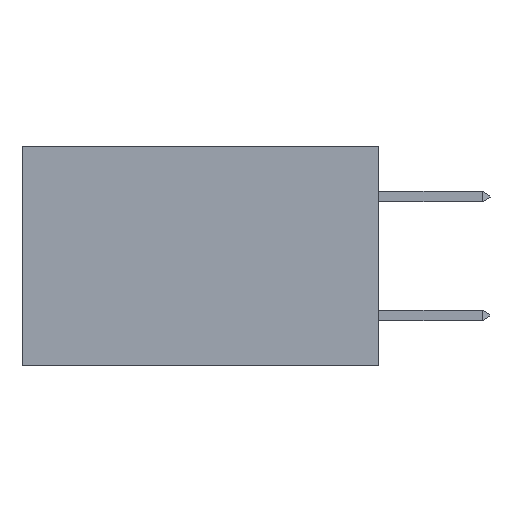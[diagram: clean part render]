
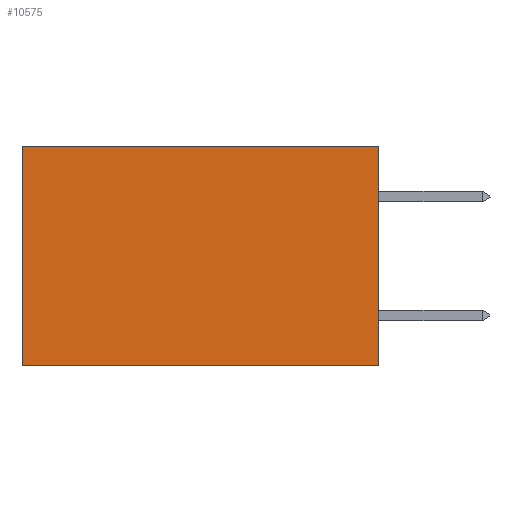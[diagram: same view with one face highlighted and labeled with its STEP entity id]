
A CAD part, left-side view. The second image highlights one B-rep face of the part: STEP entity #10575.
In plain terms, the highlighted planar face has unit normal (-1, 0, 0).
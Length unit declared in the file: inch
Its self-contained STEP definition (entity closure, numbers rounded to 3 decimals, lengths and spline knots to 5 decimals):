
#710 = ORIENTED_EDGE ( 'NONE', *, *, #22771, .F. ) ;
#1458 = VERTEX_POINT ( 'NONE', #18161 ) ;
#1689 = CARTESIAN_POINT ( 'NONE',  ( 0.2615, 0., -0.37 ) ) ;
#1898 = VERTEX_POINT ( 'NONE', #4912 ) ;
#2181 = CARTESIAN_POINT ( 'NONE',  ( 0.2615, 0., 0. ) ) ;
#3598 = LINE ( 'NONE', #21522, #13957 ) ;
#3742 = EDGE_CURVE ( 'NONE', #1898, #8556, #3598, .T. ) ;
#4210 = ORIENTED_EDGE ( 'NONE', *, *, #6669, .T. ) ;
#4297 = DIRECTION ( 'NONE',  ( 0., 1., 0. ) ) ;
#4912 = CARTESIAN_POINT ( 'NONE',  ( 0.2615, 0.6, 0. ) ) ;
#6669 = EDGE_CURVE ( 'NONE', #19979, #1898, #26027, .T. ) ;
#7958 = DIRECTION ( 'NONE',  ( 1., 0., 0. ) ) ;
#8000 = DIRECTION ( 'NONE',  ( 0., 1., 0. ) ) ;
#8039 = EDGE_LOOP ( 'NONE', ( #21949, #710, #10825, #4210 ) ) ;
#8556 = VERTEX_POINT ( 'NONE', #13973 ) ;
#8856 = VECTOR ( 'NONE', #8000, 39.37008 ) ;
#8981 = FACE_OUTER_BOUND ( 'NONE', #8039, .T. ) ;
#9508 = VECTOR ( 'NONE', #4297, 39.37008 ) ;
#10575 = ADVANCED_FACE ( 'NONE', ( #8981 ), #20424, .F. ) ;
#10825 = ORIENTED_EDGE ( 'NONE', *, *, #23929, .F. ) ;
#11150 = DIRECTION ( 'NONE',  ( 0., 0., -1. ) ) ;
#11850 = AXIS2_PLACEMENT_3D ( 'NONE', #1689, #7958, #22485 ) ;
#13017 = LINE ( 'NONE', #25884, #17910 ) ;
#13957 = VECTOR ( 'NONE', #11150, 39.37008 ) ;
#13973 = CARTESIAN_POINT ( 'NONE',  ( 0.2615, 0.6, -0.37 ) ) ;
#14990 = LINE ( 'NONE', #18356, #8856 ) ;
#15550 = DIRECTION ( 'NONE',  ( 0., 0., -1. ) ) ;
#17910 = VECTOR ( 'NONE', #15550, 39.37008 ) ;
#18161 = CARTESIAN_POINT ( 'NONE',  ( 0.2615, 0., -0.37 ) ) ;
#18356 = CARTESIAN_POINT ( 'NONE',  ( 0.2615, 0., -0.37 ) ) ;
#19979 = VERTEX_POINT ( 'NONE', #26731 ) ;
#20424 = PLANE ( 'NONE',  #11850 ) ;
#21522 = CARTESIAN_POINT ( 'NONE',  ( 0.2615, 0.6, -0.37 ) ) ;
#21949 = ORIENTED_EDGE ( 'NONE', *, *, #3742, .T. ) ;
#22485 = DIRECTION ( 'NONE',  ( 0., 0., -1. ) ) ;
#22771 = EDGE_CURVE ( 'NONE', #1458, #8556, #14990, .T. ) ;
#23929 = EDGE_CURVE ( 'NONE', #19979, #1458, #13017, .T. ) ;
#25884 = CARTESIAN_POINT ( 'NONE',  ( 0.2615, 0., -0.37 ) ) ;
#26027 = LINE ( 'NONE', #2181, #9508 ) ;
#26731 = CARTESIAN_POINT ( 'NONE',  ( 0.2615, 0., 0. ) ) ;
